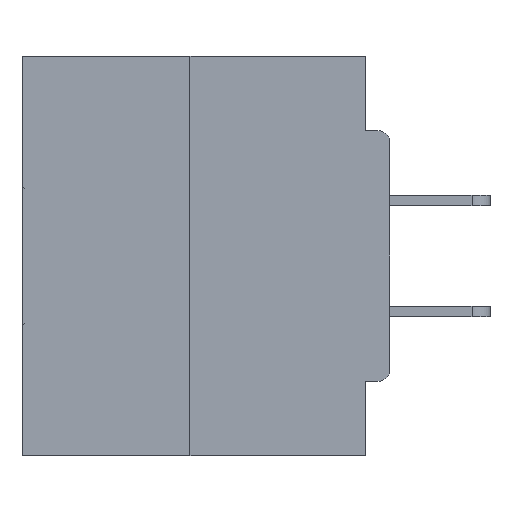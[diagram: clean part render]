
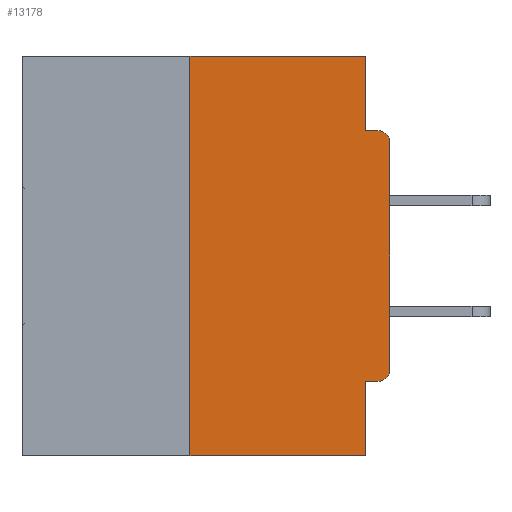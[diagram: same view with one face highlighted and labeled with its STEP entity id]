
A CAD part, left-side view. The second image highlights one B-rep face of the part: STEP entity #13178.
In plain terms, the highlighted planar face has unit normal (-1, 0, 0).
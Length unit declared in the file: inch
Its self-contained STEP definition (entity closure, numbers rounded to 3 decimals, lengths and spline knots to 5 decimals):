
#637 = VERTEX_POINT ( 'NONE', #19709 ) ;
#1726 = CARTESIAN_POINT ( 'NONE',  ( 0., 0.031, 0. ) ) ;
#1824 = CARTESIAN_POINT ( 'NONE',  ( 0., 0.015, -0.3915 ) ) ;
#1983 = CARTESIAN_POINT ( 'NONE',  ( 0., 0.031, -0.4065 ) ) ;
#2165 = DIRECTION ( 'NONE',  ( -1., 0., 0. ) ) ;
#2605 = EDGE_CURVE ( 'NONE', #15137, #29516, #12768, .T. ) ;
#3043 = LINE ( 'NONE', #13243, #18272 ) ;
#3316 = ORIENTED_EDGE ( 'NONE', *, *, #14713, .T. ) ;
#4512 = ORIENTED_EDGE ( 'NONE', *, *, #34266, .T. ) ;
#4805 = CARTESIAN_POINT ( 'NONE',  ( 0., 0.25, 0. ) ) ;
#6656 = DIRECTION ( 'NONE',  ( 0., -1., 0. ) ) ;
#7856 = LINE ( 'NONE', #38042, #14044 ) ;
#8347 = CARTESIAN_POINT ( 'NONE',  ( 0., 0., -0.4065 ) ) ;
#8363 = EDGE_CURVE ( 'NONE', #29516, #19949, #18884, .T. ) ;
#8946 = PLANE ( 'NONE',  #11978 ) ;
#10209 = ORIENTED_EDGE ( 'NONE', *, *, #33045, .F. ) ;
#10530 = VERTEX_POINT ( 'NONE', #12037 ) ;
#11978 = AXIS2_PLACEMENT_3D ( 'NONE', #30732, #18126, #30477 ) ;
#12037 = CARTESIAN_POINT ( 'NONE',  ( 0., 0.015, -0.4065 ) ) ;
#12059 = CARTESIAN_POINT ( 'NONE',  ( 0., 0., -0.1085 ) ) ;
#12567 = EDGE_LOOP ( 'NONE', ( #21545, #36810, #32843, #15997, #10209, #27044, #3316, #4512, #25295, #13670 ) ) ;
#12682 = VECTOR ( 'NONE', #38864, 39.37008 ) ;
#12768 = LINE ( 'NONE', #4805, #20916 ) ;
#12887 = VERTEX_POINT ( 'NONE', #29477 ) ;
#13178 = ADVANCED_FACE ( 'NONE', ( #30509 ), #8946, .F. ) ;
#13243 = CARTESIAN_POINT ( 'NONE',  ( 0., 0.46, -0.5 ) ) ;
#13493 = CARTESIAN_POINT ( 'NONE',  ( 0., 0.031, -0.0935 ) ) ;
#13670 = ORIENTED_EDGE ( 'NONE', *, *, #14468, .F. ) ;
#14044 = VECTOR ( 'NONE', #19720, 39.37008 ) ;
#14309 = CIRCLE ( 'NONE', #20440, 0.015 ) ;
#14351 = VECTOR ( 'NONE', #26122, 39.37008 ) ;
#14468 = EDGE_CURVE ( 'NONE', #19949, #39125, #33043, .T. ) ;
#14713 = EDGE_CURVE ( 'NONE', #31280, #21892, #21519, .T. ) ;
#15137 = VERTEX_POINT ( 'NONE', #32057 ) ;
#15334 = LINE ( 'NONE', #8347, #30686 ) ;
#15997 = ORIENTED_EDGE ( 'NONE', *, *, #36652, .F. ) ;
#16966 = DIRECTION ( 'NONE',  ( -1., 0., 0. ) ) ;
#18126 = DIRECTION ( 'NONE',  ( 1., 0., 0. ) ) ;
#18272 = VECTOR ( 'NONE', #25513, 39.37008 ) ;
#18884 = LINE ( 'NONE', #28171, #24628 ) ;
#19204 = EDGE_CURVE ( 'NONE', #15137, #12887, #3043, .T. ) ;
#19708 = CARTESIAN_POINT ( 'NONE',  ( 0., 0.031, 0. ) ) ;
#19709 = CARTESIAN_POINT ( 'NONE',  ( 0., 0.015, -0.0935 ) ) ;
#19720 = DIRECTION ( 'NONE',  ( 0., 0., -1. ) ) ;
#19864 = LINE ( 'NONE', #36040, #12682 ) ;
#19949 = VERTEX_POINT ( 'NONE', #19708 ) ;
#20440 = AXIS2_PLACEMENT_3D ( 'NONE', #1824, #16966, #38013 ) ;
#20916 = VECTOR ( 'NONE', #28817, 39.37008 ) ;
#21519 = LINE ( 'NONE', #32944, #30162 ) ;
#21545 = ORIENTED_EDGE ( 'NONE', *, *, #8363, .F. ) ;
#21892 = VERTEX_POINT ( 'NONE', #12059 ) ;
#22649 = EDGE_CURVE ( 'NONE', #10530, #31280, #14309, .T. ) ;
#24628 = VECTOR ( 'NONE', #6656, 39.37008 ) ;
#25295 = ORIENTED_EDGE ( 'NONE', *, *, #30098, .F. ) ;
#25513 = DIRECTION ( 'NONE',  ( 0., -1., 0. ) ) ;
#26122 = DIRECTION ( 'NONE',  ( 0., 0., -1. ) ) ;
#26302 = CARTESIAN_POINT ( 'NONE',  ( 0., 0.015, -0.1085 ) ) ;
#27044 = ORIENTED_EDGE ( 'NONE', *, *, #22649, .T. ) ;
#28171 = CARTESIAN_POINT ( 'NONE',  ( 0., 0.46, 0. ) ) ;
#28817 = DIRECTION ( 'NONE',  ( 0., 0., 1. ) ) ;
#29477 = CARTESIAN_POINT ( 'NONE',  ( 0., 0.031, -0.5 ) ) ;
#29516 = VERTEX_POINT ( 'NONE', #36569 ) ;
#30098 = EDGE_CURVE ( 'NONE', #39125, #637, #19864, .T. ) ;
#30162 = VECTOR ( 'NONE', #32799, 39.37008 ) ;
#30477 = DIRECTION ( 'NONE',  ( 0., 0., -1. ) ) ;
#30509 = FACE_OUTER_BOUND ( 'NONE', #12567, .T. ) ;
#30686 = VECTOR ( 'NONE', #32968, 39.37008 ) ;
#30732 = CARTESIAN_POINT ( 'NONE',  ( 0., 0.46, 0. ) ) ;
#31280 = VERTEX_POINT ( 'NONE', #37987 ) ;
#32057 = CARTESIAN_POINT ( 'NONE',  ( 0., 0.25, -0.5 ) ) ;
#32712 = AXIS2_PLACEMENT_3D ( 'NONE', #26302, #2165, #35930 ) ;
#32799 = DIRECTION ( 'NONE',  ( 0., 0., 1. ) ) ;
#32843 = ORIENTED_EDGE ( 'NONE', *, *, #19204, .T. ) ;
#32944 = CARTESIAN_POINT ( 'NONE',  ( 0., 0., 0. ) ) ;
#32968 = DIRECTION ( 'NONE',  ( 0., 1., 0. ) ) ;
#32991 = CIRCLE ( 'NONE', #32712, 0.015 ) ;
#33043 = LINE ( 'NONE', #1726, #14351 ) ;
#33045 = EDGE_CURVE ( 'NONE', #10530, #38054, #15334, .T. ) ;
#34266 = EDGE_CURVE ( 'NONE', #21892, #637, #32991, .T. ) ;
#35930 = DIRECTION ( 'NONE',  ( 0., 0., -1. ) ) ;
#36040 = CARTESIAN_POINT ( 'NONE',  ( 0., 0., -0.0935 ) ) ;
#36569 = CARTESIAN_POINT ( 'NONE',  ( 0., 0.25, 0. ) ) ;
#36652 = EDGE_CURVE ( 'NONE', #38054, #12887, #7856, .T. ) ;
#36810 = ORIENTED_EDGE ( 'NONE', *, *, #2605, .F. ) ;
#37987 = CARTESIAN_POINT ( 'NONE',  ( 0., 0., -0.3915 ) ) ;
#38013 = DIRECTION ( 'NONE',  ( 0., 0., -1. ) ) ;
#38042 = CARTESIAN_POINT ( 'NONE',  ( 0., 0.031, -0.5 ) ) ;
#38054 = VERTEX_POINT ( 'NONE', #1983 ) ;
#38864 = DIRECTION ( 'NONE',  ( 0., -1., 0. ) ) ;
#39125 = VERTEX_POINT ( 'NONE', #13493 ) ;
